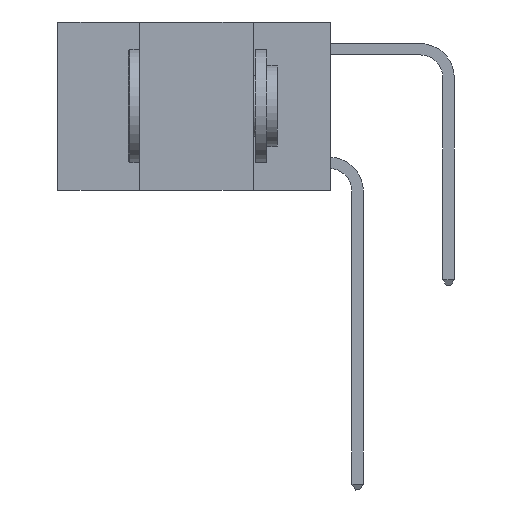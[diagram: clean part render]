
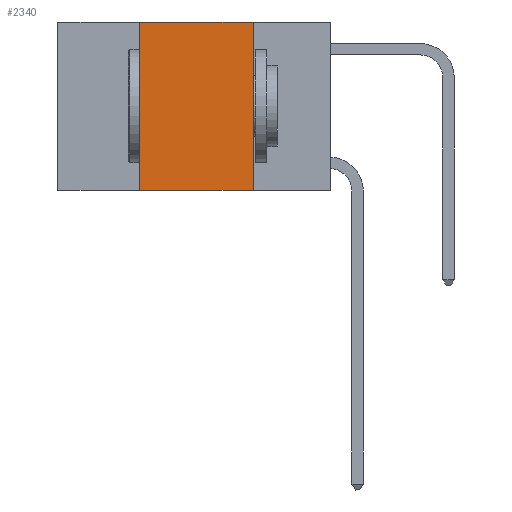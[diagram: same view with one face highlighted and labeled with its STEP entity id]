
A CAD part, left-side view. The second image highlights one B-rep face of the part: STEP entity #2340.
In plain terms, the highlighted planar face has unit normal (-1, 0, 0).
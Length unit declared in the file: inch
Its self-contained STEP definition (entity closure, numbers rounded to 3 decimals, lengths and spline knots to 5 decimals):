
#1013 = DIRECTION ( 'NONE',  ( 1., 0., 0. ) ) ;
#1617 = DIRECTION ( 'NONE',  ( 0., -1., 0. ) ) ;
#2171 = AXIS2_PLACEMENT_3D ( 'NONE', #5318, #1013, #9837 ) ;
#2340 = ADVANCED_FACE ( 'NONE', ( #14476 ), #5510, .F. ) ;
#2355 = VECTOR ( 'NONE', #1617, 39.37008 ) ;
#2678 = EDGE_CURVE ( 'NONE', #17324, #3838, #10969, .T. ) ;
#3593 = VERTEX_POINT ( 'NONE', #18562 ) ;
#3838 = VERTEX_POINT ( 'NONE', #11881 ) ;
#4205 = DIRECTION ( 'NONE',  ( 0., -1., 0. ) ) ;
#5318 = CARTESIAN_POINT ( 'NONE',  ( 0., 0.6, 0. ) ) ;
#5510 = PLANE ( 'NONE',  #2171 ) ;
#5986 = VECTOR ( 'NONE', #9340, 39.37008 ) ;
#6119 = VECTOR ( 'NONE', #14520, 39.37008 ) ;
#7856 = EDGE_CURVE ( 'NONE', #11700, #3838, #8507, .T. ) ;
#7934 = EDGE_CURVE ( 'NONE', #3593, #17324, #17686, .T. ) ;
#8507 = LINE ( 'NONE', #12934, #9717 ) ;
#8535 = LINE ( 'NONE', #8635, #6119 ) ;
#8635 = CARTESIAN_POINT ( 'NONE',  ( 0., 0.42, 0. ) ) ;
#9340 = DIRECTION ( 'NONE',  ( 0., 0., -1. ) ) ;
#9717 = VECTOR ( 'NONE', #4205, 39.37008 ) ;
#9837 = DIRECTION ( 'NONE',  ( 0., 0., -1. ) ) ;
#10859 = CARTESIAN_POINT ( 'NONE',  ( 0., 0.42, -0.37 ) ) ;
#10969 = LINE ( 'NONE', #12218, #5986 ) ;
#11057 = EDGE_LOOP ( 'NONE', ( #14219, #17354, #18102, #18757 ) ) ;
#11230 = CARTESIAN_POINT ( 'NONE',  ( 0., 0.17, 0. ) ) ;
#11700 = VERTEX_POINT ( 'NONE', #10859 ) ;
#11881 = CARTESIAN_POINT ( 'NONE',  ( 0., 0.17, -0.37 ) ) ;
#12172 = EDGE_CURVE ( 'NONE', #11700, #3593, #8535, .T. ) ;
#12218 = CARTESIAN_POINT ( 'NONE',  ( 0., 0.17, 0. ) ) ;
#12934 = CARTESIAN_POINT ( 'NONE',  ( 0., 0.6, -0.37 ) ) ;
#14219 = ORIENTED_EDGE ( 'NONE', *, *, #2678, .F. ) ;
#14476 = FACE_OUTER_BOUND ( 'NONE', #11057, .T. ) ;
#14520 = DIRECTION ( 'NONE',  ( 0., 0., 1. ) ) ;
#14689 = CARTESIAN_POINT ( 'NONE',  ( 0., 0.6, 0. ) ) ;
#17324 = VERTEX_POINT ( 'NONE', #11230 ) ;
#17354 = ORIENTED_EDGE ( 'NONE', *, *, #7934, .F. ) ;
#17686 = LINE ( 'NONE', #14689, #2355 ) ;
#18102 = ORIENTED_EDGE ( 'NONE', *, *, #12172, .F. ) ;
#18562 = CARTESIAN_POINT ( 'NONE',  ( 0., 0.42, 0. ) ) ;
#18757 = ORIENTED_EDGE ( 'NONE', *, *, #7856, .T. ) ;
